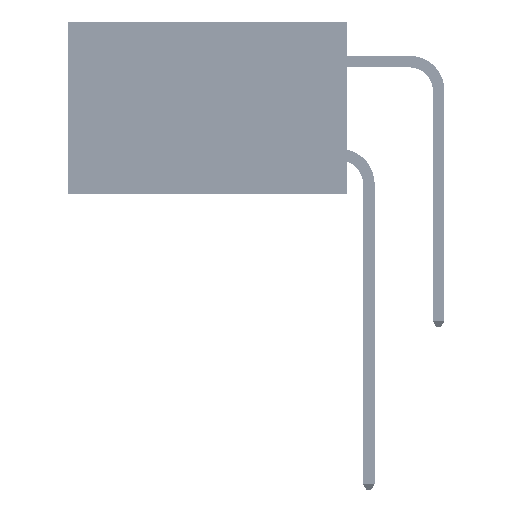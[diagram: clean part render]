
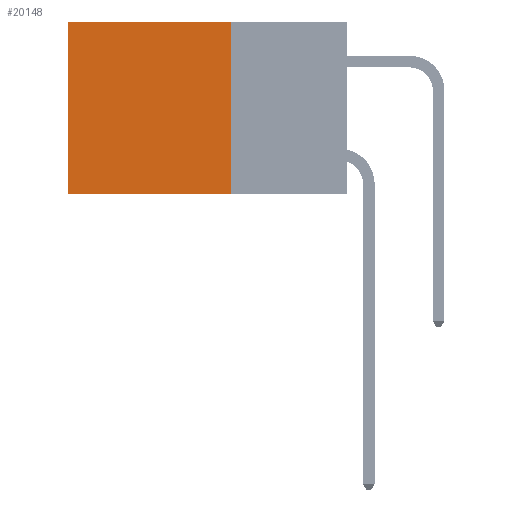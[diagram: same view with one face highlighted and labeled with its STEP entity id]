
A CAD part, left-side view. The second image highlights one B-rep face of the part: STEP entity #20148.
In plain terms, the highlighted planar face has unit normal (-1, 0, 0).
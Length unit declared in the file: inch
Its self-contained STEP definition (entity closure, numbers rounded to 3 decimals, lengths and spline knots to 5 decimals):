
#77 = CARTESIAN_POINT ( 'NONE',  ( 0.2875, 0.6, 0. ) ) ;
#299 = DIRECTION ( 'NONE',  ( 0., 1., 0. ) ) ;
#1088 = EDGE_CURVE ( 'NONE', #42151, #11200, #24766, .T. ) ;
#2200 = EDGE_CURVE ( 'NONE', #11778, #11200, #18039, .T. ) ;
#6196 = DIRECTION ( 'NONE',  ( 0., 0., -1. ) ) ;
#7249 = DIRECTION ( 'NONE',  ( 0., 0., -1. ) ) ;
#7296 = CARTESIAN_POINT ( 'NONE',  ( 0.2875, 0.25, -0.37 ) ) ;
#8928 = EDGE_LOOP ( 'NONE', ( #38208, #11852, #46283, #41733 ) ) ;
#10446 = LINE ( 'NONE', #38580, #14074 ) ;
#11020 = EDGE_CURVE ( 'NONE', #23054, #42151, #10446, .T. ) ;
#11200 = VERTEX_POINT ( 'NONE', #44616 ) ;
#11778 = VERTEX_POINT ( 'NONE', #77 ) ;
#11852 = ORIENTED_EDGE ( 'NONE', *, *, #1088, .F. ) ;
#12742 = CARTESIAN_POINT ( 'NONE',  ( 0.2875, 0.25, 0. ) ) ;
#13749 = DIRECTION ( 'NONE',  ( 0., 1., 0. ) ) ;
#14074 = VECTOR ( 'NONE', #7249, 39.37008 ) ;
#14745 = DIRECTION ( 'NONE',  ( 0., 0., -1. ) ) ;
#17434 = CARTESIAN_POINT ( 'NONE',  ( 0.2875, 0.25, 0. ) ) ;
#17781 = CARTESIAN_POINT ( 'NONE',  ( 0.2875, 0.6, 0. ) ) ;
#18039 = LINE ( 'NONE', #17781, #34095 ) ;
#18964 = FACE_OUTER_BOUND ( 'NONE', #8928, .T. ) ;
#20148 = ADVANCED_FACE ( 'NONE', ( #18964 ), #26850, .F. ) ;
#20817 = CARTESIAN_POINT ( 'NONE',  ( 0.2875, 0.25, -0.37 ) ) ;
#23054 = VERTEX_POINT ( 'NONE', #12742 ) ;
#24766 = LINE ( 'NONE', #20817, #42198 ) ;
#26850 = PLANE ( 'NONE',  #38968 ) ;
#29787 = LINE ( 'NONE', #17434, #50693 ) ;
#34095 = VECTOR ( 'NONE', #6196, 39.37008 ) ;
#35001 = DIRECTION ( 'NONE',  ( 1., 0., 0. ) ) ;
#38208 = ORIENTED_EDGE ( 'NONE', *, *, #2200, .T. ) ;
#38378 = EDGE_CURVE ( 'NONE', #23054, #11778, #29787, .T. ) ;
#38580 = CARTESIAN_POINT ( 'NONE',  ( 0.2875, 0.25, 0. ) ) ;
#38692 = CARTESIAN_POINT ( 'NONE',  ( 0.2875, 0.25, 0. ) ) ;
#38968 = AXIS2_PLACEMENT_3D ( 'NONE', #38692, #35001, #14745 ) ;
#41733 = ORIENTED_EDGE ( 'NONE', *, *, #38378, .T. ) ;
#42151 = VERTEX_POINT ( 'NONE', #7296 ) ;
#42198 = VECTOR ( 'NONE', #299, 39.37008 ) ;
#44616 = CARTESIAN_POINT ( 'NONE',  ( 0.2875, 0.6, -0.37 ) ) ;
#46283 = ORIENTED_EDGE ( 'NONE', *, *, #11020, .F. ) ;
#50693 = VECTOR ( 'NONE', #13749, 39.37008 ) ;
